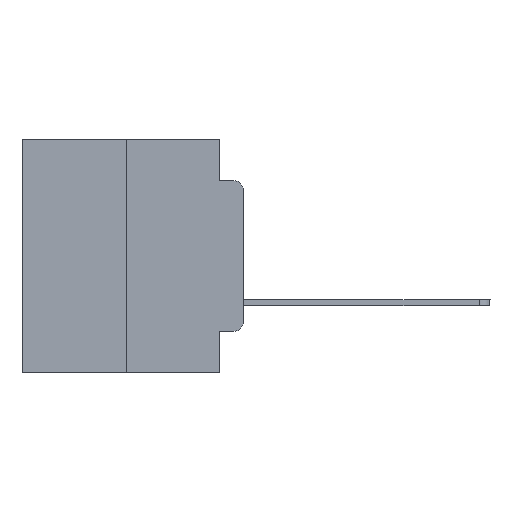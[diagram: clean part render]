
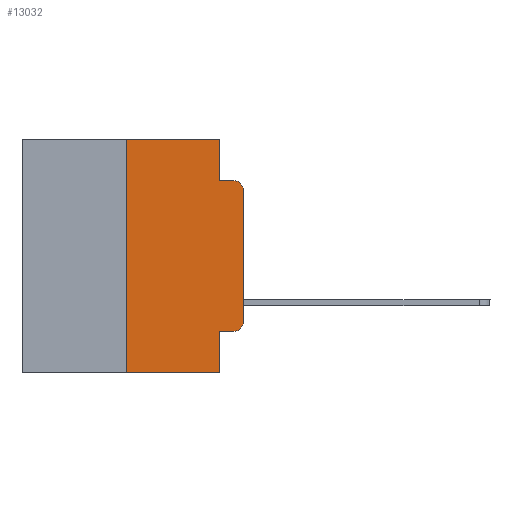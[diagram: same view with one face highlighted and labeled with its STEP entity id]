
A CAD part, left-side view. The second image highlights one B-rep face of the part: STEP entity #13032.
In plain terms, the highlighted planar face has unit normal (-1, 0, 0).
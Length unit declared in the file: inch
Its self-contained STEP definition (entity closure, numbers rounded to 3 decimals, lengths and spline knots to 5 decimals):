
#115 = VERTEX_POINT ( 'NONE', #10629 ) ;
#234 = CARTESIAN_POINT ( 'NONE',  ( 0., 0.051, 0. ) ) ;
#302 = VECTOR ( 'NONE', #21429, 39.37008 ) ;
#732 = FACE_OUTER_BOUND ( 'NONE', #2842, .T. ) ;
#964 = LINE ( 'NONE', #234, #302 ) ;
#1562 = VECTOR ( 'NONE', #12214, 39.37008 ) ;
#1762 = ORIENTED_EDGE ( 'NONE', *, *, #21986, .F. ) ;
#2048 = PLANE ( 'NONE',  #20977 ) ;
#2099 = ORIENTED_EDGE ( 'NONE', *, *, #6555, .T. ) ;
#2424 = ORIENTED_EDGE ( 'NONE', *, *, #21152, .T. ) ;
#2743 = EDGE_CURVE ( 'NONE', #19493, #14665, #14673, .T. ) ;
#2784 = VECTOR ( 'NONE', #20882, 39.37008 ) ;
#2842 = EDGE_LOOP ( 'NONE', ( #3655, #2099, #7550, #1762, #3891, #3262, #11901, #9238, #2424, #23218 ) ) ;
#3071 = VERTEX_POINT ( 'NONE', #20330 ) ;
#3262 = ORIENTED_EDGE ( 'NONE', *, *, #18023, .F. ) ;
#3328 = VECTOR ( 'NONE', #22568, 39.37008 ) ;
#3372 = VERTEX_POINT ( 'NONE', #23777 ) ;
#3655 = ORIENTED_EDGE ( 'NONE', *, *, #15849, .T. ) ;
#3789 = VERTEX_POINT ( 'NONE', #20122 ) ;
#3891 = ORIENTED_EDGE ( 'NONE', *, *, #20031, .F. ) ;
#3984 = LINE ( 'NONE', #24553, #3328 ) ;
#4101 = LINE ( 'NONE', #4644, #22865 ) ;
#4644 = CARTESIAN_POINT ( 'NONE',  ( 0., 0.473, -0.5 ) ) ;
#5081 = CARTESIAN_POINT ( 'NONE',  ( 0., 0.25, 0. ) ) ;
#6390 = AXIS2_PLACEMENT_3D ( 'NONE', #7202, #13666, #13838 ) ;
#6555 = EDGE_CURVE ( 'NONE', #115, #3789, #12895, .T. ) ;
#6639 = LINE ( 'NONE', #10459, #2784 ) ;
#7202 = CARTESIAN_POINT ( 'NONE',  ( 0., 0.02, -0.3915 ) ) ;
#7536 = CARTESIAN_POINT ( 'NONE',  ( 0., 0.051, -0.0885 ) ) ;
#7550 = ORIENTED_EDGE ( 'NONE', *, *, #17384, .F. ) ;
#7582 = VERTEX_POINT ( 'NONE', #5081 ) ;
#7587 = CARTESIAN_POINT ( 'NONE',  ( 0., 0.25, -0.5 ) ) ;
#8016 = CARTESIAN_POINT ( 'NONE',  ( 0., 0., 0. ) ) ;
#8512 = CARTESIAN_POINT ( 'NONE',  ( 0., 0.051, -0.0885 ) ) ;
#9198 = VECTOR ( 'NONE', #26510, 39.37008 ) ;
#9238 = ORIENTED_EDGE ( 'NONE', *, *, #17381, .F. ) ;
#10459 = CARTESIAN_POINT ( 'NONE',  ( 0., 0.051, 0. ) ) ;
#10629 = CARTESIAN_POINT ( 'NONE',  ( 0., 0., -0.1085 ) ) ;
#10685 = VERTEX_POINT ( 'NONE', #7536 ) ;
#11153 = DIRECTION ( 'NONE',  ( -1., 0., 0. ) ) ;
#11226 = VERTEX_POINT ( 'NONE', #21444 ) ;
#11901 = ORIENTED_EDGE ( 'NONE', *, *, #16635, .T. ) ;
#12214 = DIRECTION ( 'NONE',  ( 0., 0., 1. ) ) ;
#12826 = VECTOR ( 'NONE', #15775, 39.37008 ) ;
#12850 = LINE ( 'NONE', #8512, #23500 ) ;
#12895 = CIRCLE ( 'NONE', #23797, 0.02 ) ;
#13032 = ADVANCED_FACE ( 'NONE', ( #732 ), #2048, .F. ) ;
#13666 = DIRECTION ( 'NONE',  ( -1., 0., 0. ) ) ;
#13838 = DIRECTION ( 'NONE',  ( 0., 0., -1. ) ) ;
#14061 = LINE ( 'NONE', #20084, #9198 ) ;
#14665 = VERTEX_POINT ( 'NONE', #17341 ) ;
#14673 = CIRCLE ( 'NONE', #6390, 0.02 ) ;
#14732 = VERTEX_POINT ( 'NONE', #7587 ) ;
#15696 = LINE ( 'NONE', #22466, #12826 ) ;
#15775 = DIRECTION ( 'NONE',  ( 0., 0., 1. ) ) ;
#15849 = EDGE_CURVE ( 'NONE', #14665, #115, #18402, .T. ) ;
#16634 = DIRECTION ( 'NONE',  ( 0., -1., 0. ) ) ;
#16635 = EDGE_CURVE ( 'NONE', #14732, #11226, #4101, .T. ) ;
#17064 = DIRECTION ( 'NONE',  ( 0., 0., -1. ) ) ;
#17341 = CARTESIAN_POINT ( 'NONE',  ( 0., 0., -0.3915 ) ) ;
#17381 = EDGE_CURVE ( 'NONE', #3071, #11226, #6639, .T. ) ;
#17384 = EDGE_CURVE ( 'NONE', #10685, #3789, #12850, .T. ) ;
#18023 = EDGE_CURVE ( 'NONE', #14732, #7582, #15696, .T. ) ;
#18252 = DIRECTION ( 'NONE',  ( 1., 0., 0. ) ) ;
#18402 = LINE ( 'NONE', #8016, #1562 ) ;
#19493 = VERTEX_POINT ( 'NONE', #24534 ) ;
#20031 = EDGE_CURVE ( 'NONE', #7582, #3372, #14061, .T. ) ;
#20084 = CARTESIAN_POINT ( 'NONE',  ( 0., 0.473, 0. ) ) ;
#20122 = CARTESIAN_POINT ( 'NONE',  ( 0., 0.02, -0.0885 ) ) ;
#20240 = CARTESIAN_POINT ( 'NONE',  ( 0., 0.473, 0. ) ) ;
#20330 = CARTESIAN_POINT ( 'NONE',  ( 0., 0.051, -0.4115 ) ) ;
#20507 = DIRECTION ( 'NONE',  ( 0., 0., -1. ) ) ;
#20882 = DIRECTION ( 'NONE',  ( 0., 0., -1. ) ) ;
#20977 = AXIS2_PLACEMENT_3D ( 'NONE', #20240, #18252, #20507 ) ;
#21152 = EDGE_CURVE ( 'NONE', #3071, #19493, #3984, .T. ) ;
#21399 = CARTESIAN_POINT ( 'NONE',  ( 0., 0.02, -0.1085 ) ) ;
#21429 = DIRECTION ( 'NONE',  ( 0., 0., -1. ) ) ;
#21444 = CARTESIAN_POINT ( 'NONE',  ( 0., 0.051, -0.5 ) ) ;
#21986 = EDGE_CURVE ( 'NONE', #3372, #10685, #964, .T. ) ;
#22466 = CARTESIAN_POINT ( 'NONE',  ( 0., 0.25, 0. ) ) ;
#22568 = DIRECTION ( 'NONE',  ( 0., -1., 0. ) ) ;
#22865 = VECTOR ( 'NONE', #23272, 39.37008 ) ;
#23218 = ORIENTED_EDGE ( 'NONE', *, *, #2743, .T. ) ;
#23272 = DIRECTION ( 'NONE',  ( 0., -1., 0. ) ) ;
#23500 = VECTOR ( 'NONE', #16634, 39.37008 ) ;
#23777 = CARTESIAN_POINT ( 'NONE',  ( 0., 0.051, 0. ) ) ;
#23797 = AXIS2_PLACEMENT_3D ( 'NONE', #21399, #11153, #17064 ) ;
#24534 = CARTESIAN_POINT ( 'NONE',  ( 0., 0.02, -0.4115 ) ) ;
#24553 = CARTESIAN_POINT ( 'NONE',  ( 0., 0.051, -0.4115 ) ) ;
#26510 = DIRECTION ( 'NONE',  ( 0., -1., 0. ) ) ;
